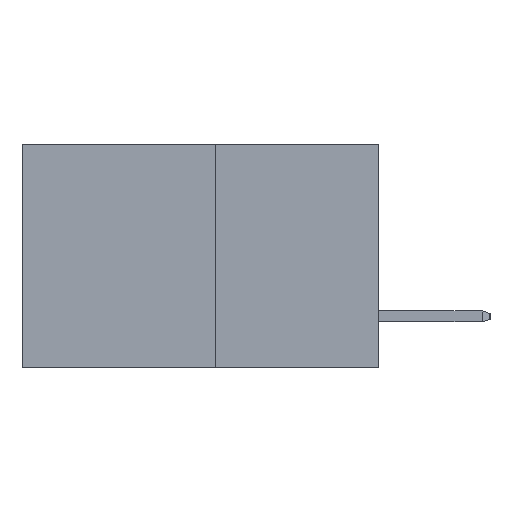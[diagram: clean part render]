
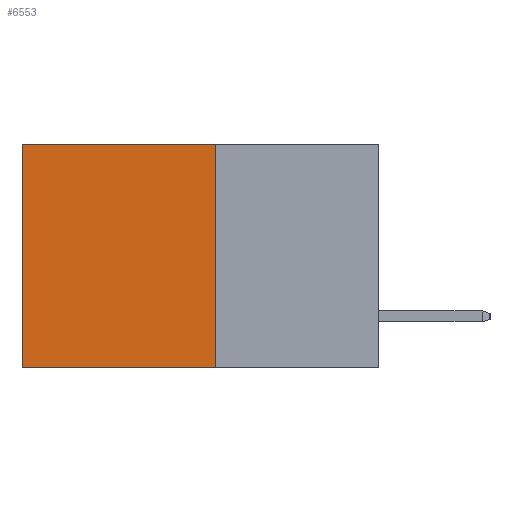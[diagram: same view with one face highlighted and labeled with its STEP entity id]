
A CAD part, left-side view. The second image highlights one B-rep face of the part: STEP entity #6553.
In plain terms, the highlighted planar face has unit normal (-1, 0, 0).
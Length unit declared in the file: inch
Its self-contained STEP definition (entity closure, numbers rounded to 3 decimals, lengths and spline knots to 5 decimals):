
#13 = EDGE_CURVE ( 'NONE', #5764, #924, #13521, .T. ) ;
#924 = VERTEX_POINT ( 'NONE', #2435 ) ;
#1831 = LINE ( 'NONE', #7635, #16004 ) ;
#2301 = ORIENTED_EDGE ( 'NONE', *, *, #7425, .F. ) ;
#2435 = CARTESIAN_POINT ( 'NONE',  ( 0.277, 0.59, 0. ) ) ;
#3117 = CARTESIAN_POINT ( 'NONE',  ( 0.277, 0.27, 0. ) ) ;
#3698 = DIRECTION ( 'NONE',  ( 0., 1., 0. ) ) ;
#3992 = ORIENTED_EDGE ( 'NONE', *, *, #13, .T. ) ;
#4810 = VECTOR ( 'NONE', #10238, 39.37008 ) ;
#5764 = VERTEX_POINT ( 'NONE', #19528 ) ;
#6553 = ADVANCED_FACE ( 'NONE', ( #17625 ), #17966, .F. ) ;
#7425 = EDGE_CURVE ( 'NONE', #23673, #22063, #1831, .T. ) ;
#7635 = CARTESIAN_POINT ( 'NONE',  ( 0.277, 0.27, -0.37 ) ) ;
#7976 = EDGE_LOOP ( 'NONE', ( #14316, #2301, #13423, #3992 ) ) ;
#9193 = VECTOR ( 'NONE', #3698, 39.37008 ) ;
#9195 = LINE ( 'NONE', #18439, #13523 ) ;
#9507 = DIRECTION ( 'NONE',  ( 0., 1., 0. ) ) ;
#10238 = DIRECTION ( 'NONE',  ( 0., 0., -1. ) ) ;
#10758 = DIRECTION ( 'NONE',  ( 0., 0., -1. ) ) ;
#11115 = AXIS2_PLACEMENT_3D ( 'NONE', #19891, #21745, #10758 ) ;
#12098 = EDGE_CURVE ( 'NONE', #5764, #23673, #19500, .T. ) ;
#13423 = ORIENTED_EDGE ( 'NONE', *, *, #12098, .F. ) ;
#13521 = LINE ( 'NONE', #3117, #9193 ) ;
#13523 = VECTOR ( 'NONE', #22120, 39.37008 ) ;
#13833 = CARTESIAN_POINT ( 'NONE',  ( 0.277, 0.27, -0.37 ) ) ;
#14316 = ORIENTED_EDGE ( 'NONE', *, *, #18754, .T. ) ;
#16004 = VECTOR ( 'NONE', #9507, 39.37008 ) ;
#16886 = CARTESIAN_POINT ( 'NONE',  ( 0.277, 0.27, -0.37 ) ) ;
#17625 = FACE_OUTER_BOUND ( 'NONE', #7976, .T. ) ;
#17966 = PLANE ( 'NONE',  #11115 ) ;
#18439 = CARTESIAN_POINT ( 'NONE',  ( 0.277, 0.59, -0.37 ) ) ;
#18754 = EDGE_CURVE ( 'NONE', #924, #22063, #9195, .T. ) ;
#19500 = LINE ( 'NONE', #13833, #4810 ) ;
#19528 = CARTESIAN_POINT ( 'NONE',  ( 0.277, 0.27, 0. ) ) ;
#19715 = CARTESIAN_POINT ( 'NONE',  ( 0.277, 0.59, -0.37 ) ) ;
#19891 = CARTESIAN_POINT ( 'NONE',  ( 0.277, 0.27, -0.37 ) ) ;
#21745 = DIRECTION ( 'NONE',  ( 1., 0., 0. ) ) ;
#22063 = VERTEX_POINT ( 'NONE', #19715 ) ;
#22120 = DIRECTION ( 'NONE',  ( 0., 0., -1. ) ) ;
#23673 = VERTEX_POINT ( 'NONE', #16886 ) ;
